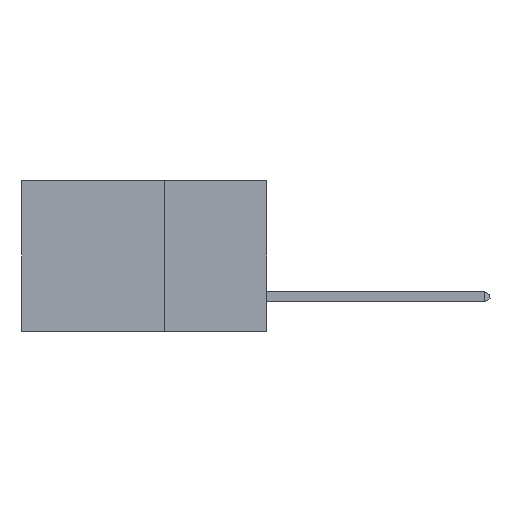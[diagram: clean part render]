
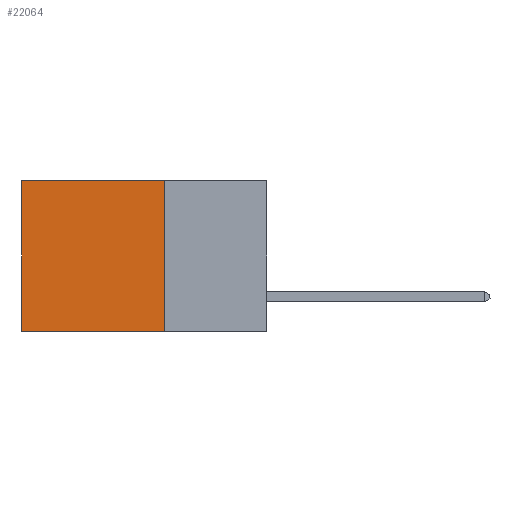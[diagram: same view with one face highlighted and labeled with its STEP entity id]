
A CAD part, left-side view. The second image highlights one B-rep face of the part: STEP entity #22064.
In plain terms, the highlighted planar face has unit normal (-1, 0, 0).
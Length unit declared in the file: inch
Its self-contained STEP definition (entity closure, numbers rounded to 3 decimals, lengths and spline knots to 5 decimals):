
#19 = CARTESIAN_POINT ( 'NONE',  ( 0.2875, 0.25, -0.37 ) ) ;
#983 = EDGE_CURVE ( 'NONE', #13884, #3058, #17465, .T. ) ;
#1860 = VECTOR ( 'NONE', #15519, 39.37008 ) ;
#2565 = ORIENTED_EDGE ( 'NONE', *, *, #983, .F. ) ;
#2576 = EDGE_LOOP ( 'NONE', ( #19938, #2565, #19343, #20646 ) ) ;
#3058 = VERTEX_POINT ( 'NONE', #21751 ) ;
#3168 = EDGE_CURVE ( 'NONE', #21430, #13884, #7259, .T. ) ;
#3618 = CARTESIAN_POINT ( 'NONE',  ( 0.2875, 0.25, -0.37 ) ) ;
#3622 = EDGE_CURVE ( 'NONE', #21069, #3058, #21603, .T. ) ;
#7259 = LINE ( 'NONE', #21217, #21624 ) ;
#7302 = DIRECTION ( 'NONE',  ( 1., 0., 0. ) ) ;
#9118 = PLANE ( 'NONE',  #16692 ) ;
#11582 = CARTESIAN_POINT ( 'NONE',  ( 0.2875, 0.6, 0. ) ) ;
#12761 = FACE_OUTER_BOUND ( 'NONE', #2576, .T. ) ;
#13884 = VERTEX_POINT ( 'NONE', #19 ) ;
#14508 = CARTESIAN_POINT ( 'NONE',  ( 0.2875, 0.25, 0. ) ) ;
#14864 = EDGE_CURVE ( 'NONE', #21430, #21069, #16072, .T. ) ;
#15486 = VECTOR ( 'NONE', #15644, 39.37008 ) ;
#15519 = DIRECTION ( 'NONE',  ( 0., 1., 0. ) ) ;
#15594 = DIRECTION ( 'NONE',  ( 0., 0., -1. ) ) ;
#15644 = DIRECTION ( 'NONE',  ( 0., 1., 0. ) ) ;
#15708 = CARTESIAN_POINT ( 'NONE',  ( 0.2875, 0.6, 0. ) ) ;
#16072 = LINE ( 'NONE', #21194, #15486 ) ;
#16692 = AXIS2_PLACEMENT_3D ( 'NONE', #18553, #7302, #20427 ) ;
#17465 = LINE ( 'NONE', #3618, #1860 ) ;
#18553 = CARTESIAN_POINT ( 'NONE',  ( 0.2875, 0.25, 0. ) ) ;
#19343 = ORIENTED_EDGE ( 'NONE', *, *, #3168, .F. ) ;
#19938 = ORIENTED_EDGE ( 'NONE', *, *, #3622, .T. ) ;
#20427 = DIRECTION ( 'NONE',  ( 0., 0., -1. ) ) ;
#20646 = ORIENTED_EDGE ( 'NONE', *, *, #14864, .T. ) ;
#20803 = DIRECTION ( 'NONE',  ( 0., 0., -1. ) ) ;
#21038 = VECTOR ( 'NONE', #15594, 39.37008 ) ;
#21069 = VERTEX_POINT ( 'NONE', #11582 ) ;
#21194 = CARTESIAN_POINT ( 'NONE',  ( 0.2875, 0.25, 0. ) ) ;
#21217 = CARTESIAN_POINT ( 'NONE',  ( 0.2875, 0.25, 0. ) ) ;
#21430 = VERTEX_POINT ( 'NONE', #14508 ) ;
#21603 = LINE ( 'NONE', #15708, #21038 ) ;
#21624 = VECTOR ( 'NONE', #20803, 39.37008 ) ;
#21751 = CARTESIAN_POINT ( 'NONE',  ( 0.2875, 0.6, -0.37 ) ) ;
#22064 = ADVANCED_FACE ( 'NONE', ( #12761 ), #9118, .F. ) ;
